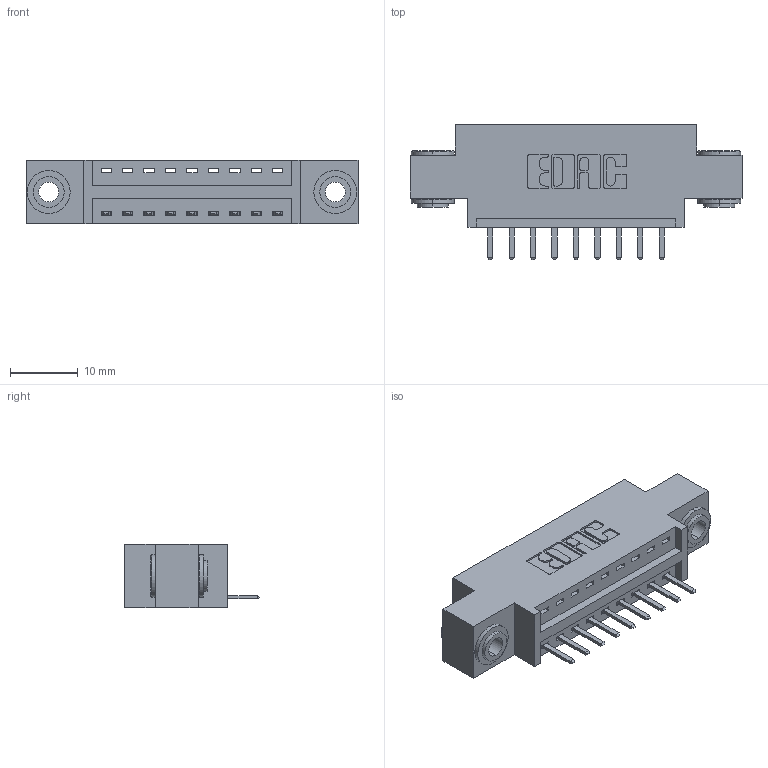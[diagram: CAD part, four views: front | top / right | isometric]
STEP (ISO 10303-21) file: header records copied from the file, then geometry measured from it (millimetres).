
FILE_DESCRIPTION (( 'STEP AP203' ), '1' );
FILE_NAME ('346-009-520-603.STEP', '2022-05-04T22:00:27', ( '' ), ( '' ), 'SwSTEP 2.0', 'SolidWorks 2020', '' );
FILE_SCHEMA (( 'CONFIG_CONTROL_DESIGN' ));
Length unit declared in the file: inch
Products named in the file (4): 345-250-002_345-250-002-102; 346 Part_0.170 Offset - 0.156 Dia-TH; 346-009-520-603; 345-292-001_345-293-120
Assembly tree (12 placements, depth 2):
  346-009-520-603
    346 Part_0.170 Offset - 0.156 Dia-TH
    345-292-001_345-293-120  x9
    345-250-002_345-250-002-102  x2
Bounding box: 49.15 x 20.02 x 9.4 mm (x, y, z)
Volume: 4298.1 mm3; surface area: 5341.3 mm2
Topology: 12 solids, 12 shells, 736 faces, 2109 edges, 1378 vertices
Faces by surface type: plane 482, cylinder 246, cone 8
Entity records: 11340 total; most frequent: CARTESIAN_POINT 1948, ORIENTED_EDGE 1870, DIRECTION 1775, EDGE_CURVE 935, LINE 739, VECTOR 739, VERTEX_POINT 618, AXIS2_PLACEMENT_3D 518
